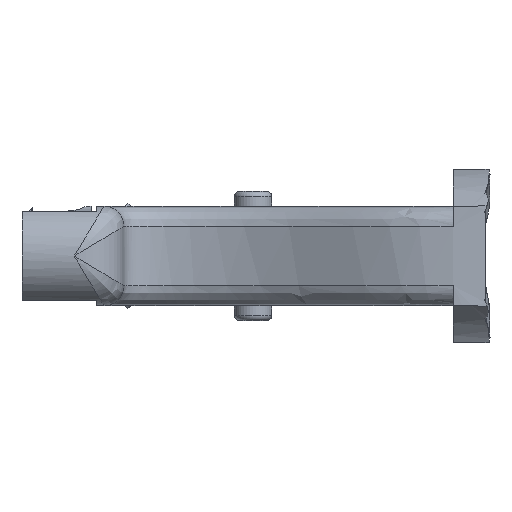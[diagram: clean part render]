
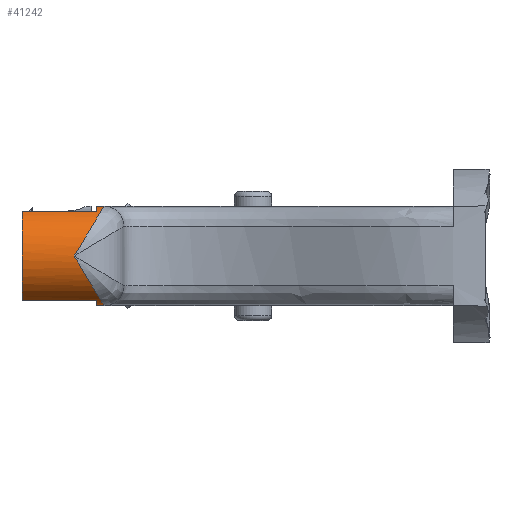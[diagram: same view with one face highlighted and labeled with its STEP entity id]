
A CAD part, left-side view. The second image highlights one B-rep face of the part: STEP entity #41242.
In plain terms, the highlighted cylindrical face has radius 10 mm (diameter 20 mm), a partial arc.
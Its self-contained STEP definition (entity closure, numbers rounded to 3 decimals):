
#142=CYLINDRICAL_SURFACE('',#42116,10.);
#727=B_SPLINE_CURVE_WITH_KNOTS('',3,(#86165,#86166,#86167,#86168,#86169,
#86170,#86171,#86172,#86173,#86174,#86175,#86176,#86177,#86178,#86179,#86180,
#86181,#86182,#86183,#86184,#86185,#86186,#86187,#86188),.UNSPECIFIED.,
 .F.,.F.,(4,3,3,2,3,3,3,3,4),(4.712,4.909,5.105,5.301,
5.498,5.694,5.89,6.087,6.283),
 .UNSPECIFIED.);
#729=B_SPLINE_CURVE_WITH_KNOTS('',3,(#86215,#86216,#86217,#86218,#86219,
#86220,#86221,#86222,#86223,#86224,#86225,#86226,#86227,#86228,#86229,#86230,
#86231,#86232,#86233,#86234,#86235,#86236,#86237,#86238),.UNSPECIFIED.,
 .F.,.F.,(4,2,3,3,3,3,3,3,4),(0.,0.196,0.393,0.589,0.785,
0.982,1.178,1.374,1.571),.UNSPECIFIED.);
#1041=CIRCLE('',#41748,10.);
#1083=CIRCLE('',#41844,10.);
#1155=CIRCLE('',#42095,10.);
#3943=FACE_OUTER_BOUND('',#6275,.T.);
#6275=EDGE_LOOP('',(#37267,#37268,#37269,#37270,#37271,#37272,#37273,#37274,
#37275));
#8510=LINE('',#76797,#11315);
#8579=LINE('',#77651,#11384);
#8655=LINE('',#78162,#11460);
#9116=LINE('',#86065,#11921);
#11315=VECTOR('',#44968,1.5);
#11384=VECTOR('',#45135,1.5);
#11460=VECTOR('',#45287,15.);
#11921=VECTOR('',#46452,15.);
#18112=VERTEX_POINT('',#76794);
#18113=VERTEX_POINT('',#76796);
#18229=VERTEX_POINT('',#77648);
#18230=VERTEX_POINT('',#77650);
#18312=VERTEX_POINT('',#78160);
#18313=VERTEX_POINT('',#78161);
#18454=VERTEX_POINT('',#80467);
#18765=VERTEX_POINT('',#86059);
#18768=VERTEX_POINT('',#86140);
#24021=EDGE_CURVE('',#18112,#18113,#8510,.T.);
#24150=EDGE_CURVE('',#18229,#18230,#8579,.T.);
#24254=EDGE_CURVE('',#18312,#18313,#8655,.T.);
#24260=EDGE_CURVE('',#18113,#18312,#1041,.T.);
#24459=EDGE_CURVE('',#18313,#18454,#1083,.T.);
#24980=EDGE_CURVE('',#18765,#18229,#1155,.T.);
#24983=EDGE_CURVE('',#18454,#18765,#9116,.T.);
#24995=EDGE_CURVE('',#18768,#18230,#727,.T.);
#24997=EDGE_CURVE('',#18112,#18768,#729,.T.);
#37267=ORIENTED_EDGE('',*,*,#24983,.F.);
#37268=ORIENTED_EDGE('',*,*,#24459,.F.);
#37269=ORIENTED_EDGE('',*,*,#24254,.F.);
#37270=ORIENTED_EDGE('',*,*,#24260,.F.);
#37271=ORIENTED_EDGE('',*,*,#24021,.F.);
#37272=ORIENTED_EDGE('',*,*,#24997,.T.);
#37273=ORIENTED_EDGE('',*,*,#24995,.T.);
#37274=ORIENTED_EDGE('',*,*,#24150,.F.);
#37275=ORIENTED_EDGE('',*,*,#24980,.F.);
#41242=ADVANCED_FACE('',(#3943),#142,.T.);
#41748=AXIS2_PLACEMENT_3D('',#78271,#45296,#45297);
#41844=AXIS2_PLACEMENT_3D('',#80468,#45586,#45587);
#42095=AXIS2_PLACEMENT_3D('',#86061,#46446,#46447);
#42116=AXIS2_PLACEMENT_3D('',#86214,#46497,#46498);
#44968=DIRECTION('',(0.,1.,0.));
#45135=DIRECTION('',(0.,-1.,0.));
#45287=DIRECTION('',(0.,1.,0.));
#45296=DIRECTION('center_axis',(0.,1.,0.));
#45297=DIRECTION('ref_axis',(0.,0.,-1.));
#45586=DIRECTION('center_axis',(0.,1.,0.));
#45587=DIRECTION('ref_axis',(0.,0.,-1.));
#46446=DIRECTION('center_axis',(0.,1.,0.));
#46447=DIRECTION('ref_axis',(0.,0.,-1.));
#46452=DIRECTION('',(0.,-1.,0.));
#46497=DIRECTION('center_axis',(0.,-1.,0.));
#46498=DIRECTION('ref_axis',(0.,0.,-1.));
#76794=CARTESIAN_POINT('',(-85.,31.,7.5));
#76796=CARTESIAN_POINT('',(-85.,32.5,7.5));
#76797=CARTESIAN_POINT('',(-85.,31.,7.5));
#77648=CARTESIAN_POINT('',(-85.,32.5,27.5));
#77650=CARTESIAN_POINT('',(-85.,31.,27.5));
#77651=CARTESIAN_POINT('',(-85.,32.5,27.5));
#78160=CARTESIAN_POINT('',(-89.359,32.5,8.5));
#78161=CARTESIAN_POINT('',(-89.359,47.5,8.5));
#78162=CARTESIAN_POINT('',(-89.359,32.5,8.5));
#78271=CARTESIAN_POINT('Origin',(-85.,32.5,17.5));
#80467=CARTESIAN_POINT('',(-89.359,47.5,26.5));
#80468=CARTESIAN_POINT('Origin',(-85.,47.5,17.5));
#86059=CARTESIAN_POINT('',(-89.359,32.5,26.5));
#86061=CARTESIAN_POINT('Origin',(-85.,32.5,17.5));
#86065=CARTESIAN_POINT('',(-89.359,47.5,26.5));
#86140=CARTESIAN_POINT('',(-95.,37.,17.5));
#86165=CARTESIAN_POINT('Ctrl Pts',(-95.,37.,17.5));
#86166=CARTESIAN_POINT('Ctrl Pts',(-95.,36.646,18.089));
#86167=CARTESIAN_POINT('Ctrl Pts',(-94.947,36.278,18.703));
#86168=CARTESIAN_POINT('Ctrl Pts',(-94.832,35.905,19.325));
#86169=CARTESIAN_POINT('Ctrl Pts',(-94.717,35.532,19.946));
#86170=CARTESIAN_POINT('Ctrl Pts',(-94.539,35.155,20.575));
#86171=CARTESIAN_POINT('Ctrl Pts',(-94.294,34.786,21.19));
#86172=CARTESIAN_POINT('Ctrl Pts',(-94.05,34.416,21.806));
#86173=CARTESIAN_POINT('Ctrl Pts',(-93.739,34.054,22.409));
#86174=CARTESIAN_POINT('Ctrl Pts',(-92.992,33.371,23.549));
#86175=CARTESIAN_POINT('Ctrl Pts',(-92.557,33.049,24.085));
#86176=CARTESIAN_POINT('Ctrl Pts',(-92.071,32.757,24.571));
#86177=CARTESIAN_POINT('Ctrl Pts',(-91.585,32.466,25.057));
#86178=CARTESIAN_POINT('Ctrl Pts',(-91.049,32.205,25.492));
#86179=CARTESIAN_POINT('Ctrl Pts',(-90.479,31.981,25.865));
#86180=CARTESIAN_POINT('Ctrl Pts',(-89.91,31.757,26.238));
#86181=CARTESIAN_POINT('Ctrl Pts',(-89.307,31.57,26.549));
#86182=CARTESIAN_POINT('Ctrl Pts',(-88.691,31.424,26.794));
#86183=CARTESIAN_POINT('Ctrl Pts',(-88.075,31.277,27.039));
#86184=CARTESIAN_POINT('Ctrl Pts',(-87.446,31.17,27.217));
#86185=CARTESIAN_POINT('Ctrl Pts',(-86.825,31.101,27.332));
#86186=CARTESIAN_POINT('Ctrl Pts',(-86.203,31.032,27.447));
#86187=CARTESIAN_POINT('Ctrl Pts',(-85.589,31.,27.5));
#86188=CARTESIAN_POINT('Ctrl Pts',(-85.,31.,27.5));
#86214=CARTESIAN_POINT('Origin',(-85.,31.,17.5));
#86215=CARTESIAN_POINT('Ctrl Pts',(-85.,31.,7.5));
#86216=CARTESIAN_POINT('Ctrl Pts',(-85.589,31.,7.5));
#86217=CARTESIAN_POINT('Ctrl Pts',(-86.203,31.032,7.553));
#86218=CARTESIAN_POINT('Ctrl Pts',(-87.446,31.17,7.783));
#86219=CARTESIAN_POINT('Ctrl Pts',(-88.075,31.277,7.961));
#86220=CARTESIAN_POINT('Ctrl Pts',(-88.691,31.424,8.206));
#86221=CARTESIAN_POINT('Ctrl Pts',(-89.307,31.57,8.451));
#86222=CARTESIAN_POINT('Ctrl Pts',(-89.91,31.757,8.762));
#86223=CARTESIAN_POINT('Ctrl Pts',(-90.479,31.981,9.135));
#86224=CARTESIAN_POINT('Ctrl Pts',(-91.049,32.205,9.508));
#86225=CARTESIAN_POINT('Ctrl Pts',(-91.585,32.466,9.943));
#86226=CARTESIAN_POINT('Ctrl Pts',(-92.071,32.757,10.429));
#86227=CARTESIAN_POINT('Ctrl Pts',(-92.557,33.049,10.915));
#86228=CARTESIAN_POINT('Ctrl Pts',(-92.992,33.371,11.451));
#86229=CARTESIAN_POINT('Ctrl Pts',(-93.366,33.713,12.021));
#86230=CARTESIAN_POINT('Ctrl Pts',(-93.739,34.054,12.591));
#86231=CARTESIAN_POINT('Ctrl Pts',(-94.05,34.416,13.194));
#86232=CARTESIAN_POINT('Ctrl Pts',(-94.294,34.786,13.81));
#86233=CARTESIAN_POINT('Ctrl Pts',(-94.539,35.155,14.425));
#86234=CARTESIAN_POINT('Ctrl Pts',(-94.717,35.532,15.054));
#86235=CARTESIAN_POINT('Ctrl Pts',(-94.832,35.905,15.675));
#86236=CARTESIAN_POINT('Ctrl Pts',(-94.947,36.278,16.297));
#86237=CARTESIAN_POINT('Ctrl Pts',(-95.,36.646,16.911));
#86238=CARTESIAN_POINT('Ctrl Pts',(-95.,37.,17.5));
